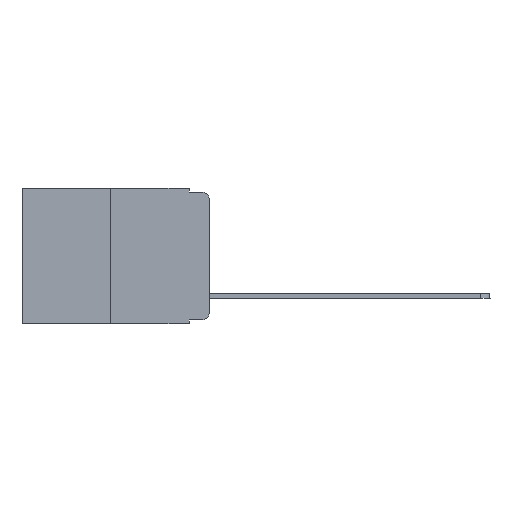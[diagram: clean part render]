
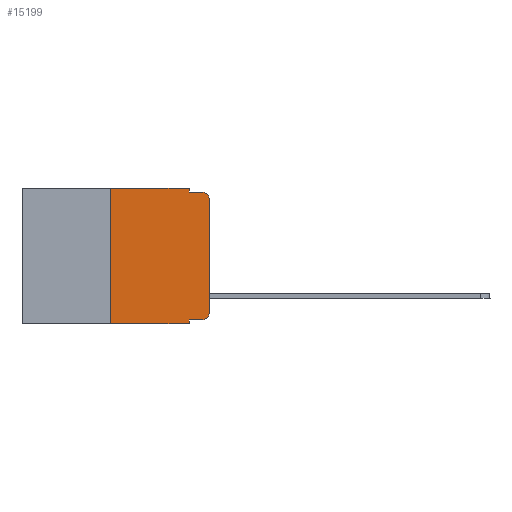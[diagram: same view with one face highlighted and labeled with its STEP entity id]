
A CAD part, left-side view. The second image highlights one B-rep face of the part: STEP entity #15199.
In plain terms, the highlighted planar face has unit normal (-1, 0, 0).
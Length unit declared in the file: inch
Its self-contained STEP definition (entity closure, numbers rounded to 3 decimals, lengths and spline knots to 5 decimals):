
#123 = VECTOR ( 'NONE', #6496, 39.37008 ) ;
#335 = ORIENTED_EDGE ( 'NONE', *, *, #609, .F. ) ;
#609 = EDGE_CURVE ( 'NONE', #7783, #2002, #6020, .T. ) ;
#617 = CIRCLE ( 'NONE', #929, 0.02 ) ;
#821 = CARTESIAN_POINT ( 'NONE',  ( 0., 0.02, -0.03 ) ) ;
#929 = AXIS2_PLACEMENT_3D ( 'NONE', #5383, #14076, #7228 ) ;
#1051 = EDGE_CURVE ( 'NONE', #7811, #11009, #12037, .T. ) ;
#1073 = PLANE ( 'NONE',  #17217 ) ;
#1154 = DIRECTION ( 'NONE',  ( 1., 0., 0. ) ) ;
#1168 = ORIENTED_EDGE ( 'NONE', *, *, #20416, .F. ) ;
#1578 = ORIENTED_EDGE ( 'NONE', *, *, #13036, .T. ) ;
#1686 = VECTOR ( 'NONE', #9570, 39.37008 ) ;
#1929 = LINE ( 'NONE', #2751, #1686 ) ;
#2002 = VERTEX_POINT ( 'NONE', #7484 ) ;
#2336 = CARTESIAN_POINT ( 'NONE',  ( 0., 0.051, 0. ) ) ;
#2645 = CARTESIAN_POINT ( 'NONE',  ( 0., 0.25, 0. ) ) ;
#2751 = CARTESIAN_POINT ( 'NONE',  ( 0., 0., 0. ) ) ;
#2753 = ORIENTED_EDGE ( 'NONE', *, *, #11002, .T. ) ;
#2944 = DIRECTION ( 'NONE',  ( 0., 0., -1. ) ) ;
#3010 = CARTESIAN_POINT ( 'NONE',  ( 0., 0.25, 0. ) ) ;
#3016 = EDGE_CURVE ( 'NONE', #10652, #2002, #13406, .T. ) ;
#3284 = EDGE_CURVE ( 'NONE', #17698, #7811, #5666, .T. ) ;
#4046 = VECTOR ( 'NONE', #22375, 39.37008 ) ;
#4529 = AXIS2_PLACEMENT_3D ( 'NONE', #821, #9753, #7835 ) ;
#4571 = VERTEX_POINT ( 'NONE', #19465 ) ;
#5383 = CARTESIAN_POINT ( 'NONE',  ( 0., 0.02, -0.313 ) ) ;
#5666 = LINE ( 'NONE', #2645, #18604 ) ;
#5673 = VECTOR ( 'NONE', #13010, 39.37008 ) ;
#5872 = ORIENTED_EDGE ( 'NONE', *, *, #15208, .T. ) ;
#6020 = LINE ( 'NONE', #18360, #15374 ) ;
#6097 = DIRECTION ( 'NONE',  ( 0., 0., 1. ) ) ;
#6332 = CARTESIAN_POINT ( 'NONE',  ( 0., 0.473, 0. ) ) ;
#6400 = CARTESIAN_POINT ( 'NONE',  ( 0., 0.473, 0. ) ) ;
#6496 = DIRECTION ( 'NONE',  ( 0., 0., -1. ) ) ;
#6627 = VERTEX_POINT ( 'NONE', #11455 ) ;
#6795 = ORIENTED_EDGE ( 'NONE', *, *, #8726, .F. ) ;
#7228 = DIRECTION ( 'NONE',  ( 0., 0., -1. ) ) ;
#7484 = CARTESIAN_POINT ( 'NONE',  ( 0., 0.02, -0.01 ) ) ;
#7783 = VERTEX_POINT ( 'NONE', #17152 ) ;
#7811 = VERTEX_POINT ( 'NONE', #3010 ) ;
#7835 = DIRECTION ( 'NONE',  ( 0., 0., -1. ) ) ;
#8015 = EDGE_CURVE ( 'NONE', #17698, #17932, #20048, .T. ) ;
#8083 = VECTOR ( 'NONE', #11550, 39.37008 ) ;
#8726 = EDGE_CURVE ( 'NONE', #11009, #7783, #18611, .T. ) ;
#8738 = CARTESIAN_POINT ( 'NONE',  ( 0., 0.473, -0.343 ) ) ;
#9570 = DIRECTION ( 'NONE',  ( 0., 0., 1. ) ) ;
#9729 = LINE ( 'NONE', #11766, #8083 ) ;
#9753 = DIRECTION ( 'NONE',  ( -1., 0., 0. ) ) ;
#10652 = VERTEX_POINT ( 'NONE', #22116 ) ;
#11002 = EDGE_CURVE ( 'NONE', #4571, #19364, #617, .T. ) ;
#11009 = VERTEX_POINT ( 'NONE', #19362 ) ;
#11455 = CARTESIAN_POINT ( 'NONE',  ( 0., 0.051, -0.333 ) ) ;
#11550 = DIRECTION ( 'NONE',  ( 0., -1., 0. ) ) ;
#11707 = LINE ( 'NONE', #17250, #123 ) ;
#11766 = CARTESIAN_POINT ( 'NONE',  ( 0., 0.051, -0.333 ) ) ;
#12037 = LINE ( 'NONE', #6332, #4046 ) ;
#13010 = DIRECTION ( 'NONE',  ( 0., 0., -1. ) ) ;
#13036 = EDGE_CURVE ( 'NONE', #19364, #10652, #1929, .T. ) ;
#13312 = ORIENTED_EDGE ( 'NONE', *, *, #8015, .T. ) ;
#13406 = CIRCLE ( 'NONE', #4529, 0.02 ) ;
#13656 = ORIENTED_EDGE ( 'NONE', *, *, #3284, .F. ) ;
#14076 = DIRECTION ( 'NONE',  ( -1., 0., 0. ) ) ;
#14397 = FACE_OUTER_BOUND ( 'NONE', #21220, .T. ) ;
#15199 = ADVANCED_FACE ( 'NONE', ( #14397 ), #1073, .F. ) ;
#15208 = EDGE_CURVE ( 'NONE', #6627, #4571, #9729, .T. ) ;
#15374 = VECTOR ( 'NONE', #21756, 39.37008 ) ;
#16050 = ORIENTED_EDGE ( 'NONE', *, *, #1051, .F. ) ;
#16134 = CARTESIAN_POINT ( 'NONE',  ( 0., 0.051, -0.343 ) ) ;
#16492 = VECTOR ( 'NONE', #19416, 39.37008 ) ;
#17152 = CARTESIAN_POINT ( 'NONE',  ( 0., 0.051, -0.01 ) ) ;
#17217 = AXIS2_PLACEMENT_3D ( 'NONE', #6400, #1154, #2944 ) ;
#17250 = CARTESIAN_POINT ( 'NONE',  ( 0., 0.051, 0. ) ) ;
#17459 = ORIENTED_EDGE ( 'NONE', *, *, #3016, .T. ) ;
#17698 = VERTEX_POINT ( 'NONE', #22458 ) ;
#17932 = VERTEX_POINT ( 'NONE', #16134 ) ;
#18360 = CARTESIAN_POINT ( 'NONE',  ( 0., 0.051, -0.01 ) ) ;
#18604 = VECTOR ( 'NONE', #6097, 39.37008 ) ;
#18611 = LINE ( 'NONE', #2336, #5673 ) ;
#19362 = CARTESIAN_POINT ( 'NONE',  ( 0., 0.051, 0. ) ) ;
#19364 = VERTEX_POINT ( 'NONE', #19635 ) ;
#19416 = DIRECTION ( 'NONE',  ( 0., -1., 0. ) ) ;
#19465 = CARTESIAN_POINT ( 'NONE',  ( 0., 0.02, -0.333 ) ) ;
#19635 = CARTESIAN_POINT ( 'NONE',  ( 0., 0., -0.313 ) ) ;
#20048 = LINE ( 'NONE', #8738, #16492 ) ;
#20416 = EDGE_CURVE ( 'NONE', #6627, #17932, #11707, .T. ) ;
#21220 = EDGE_LOOP ( 'NONE', ( #1578, #17459, #335, #6795, #16050, #13656, #13312, #1168, #5872, #2753 ) ) ;
#21756 = DIRECTION ( 'NONE',  ( 0., -1., 0. ) ) ;
#22116 = CARTESIAN_POINT ( 'NONE',  ( 0., 0., -0.03 ) ) ;
#22375 = DIRECTION ( 'NONE',  ( 0., -1., 0. ) ) ;
#22458 = CARTESIAN_POINT ( 'NONE',  ( 0., 0.25, -0.343 ) ) ;
